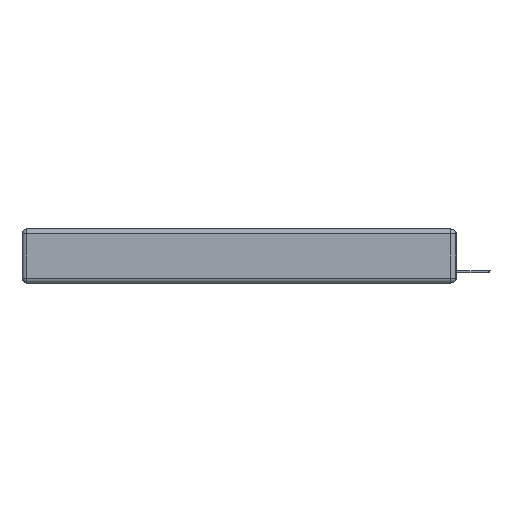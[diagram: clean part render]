
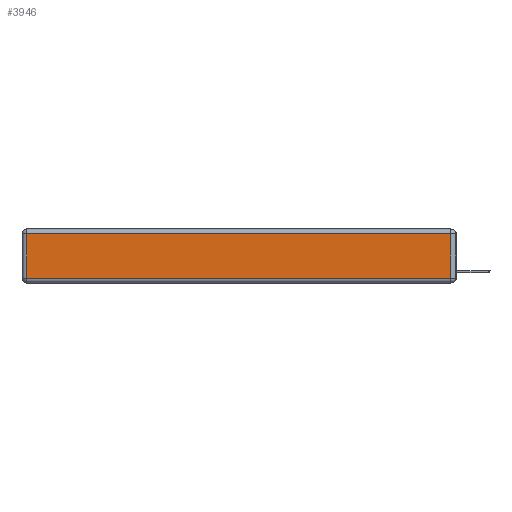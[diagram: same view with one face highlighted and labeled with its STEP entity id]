
A CAD part, left-side view. The second image highlights one B-rep face of the part: STEP entity #3946.
In plain terms, the highlighted planar face has unit normal (-1, 0, 0).
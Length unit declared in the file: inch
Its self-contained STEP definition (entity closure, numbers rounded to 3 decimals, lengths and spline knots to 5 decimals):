
#517 = DIRECTION ( 'NONE',  ( 0., 1., 0. ) ) ;
#1067 = VERTEX_POINT ( 'NONE', #14032 ) ;
#1419 = EDGE_LOOP ( 'NONE', ( #9981, #1592, #5271, #12436 ) ) ;
#1592 = ORIENTED_EDGE ( 'NONE', *, *, #12692, .T. ) ;
#1711 = EDGE_CURVE ( 'NONE', #8032, #10119, #11388, .T. ) ;
#3587 = LINE ( 'NONE', #9226, #16552 ) ;
#3635 = CARTESIAN_POINT ( 'NONE',  ( 0., 2.72, -0.03 ) ) ;
#3847 = CARTESIAN_POINT ( 'NONE',  ( 0., 0.03, -0.313 ) ) ;
#3946 = ADVANCED_FACE ( 'NONE', ( #14470 ), #17246, .T. ) ;
#4474 = EDGE_CURVE ( 'NONE', #1067, #8032, #13152, .T. ) ;
#4780 = DIRECTION ( 'NONE',  ( 0., -1., 0. ) ) ;
#5271 = ORIENTED_EDGE ( 'NONE', *, *, #4474, .T. ) ;
#5596 = VECTOR ( 'NONE', #517, 39.37008 ) ;
#5714 = EDGE_CURVE ( 'NONE', #10119, #10788, #12902, .T. ) ;
#5814 = CARTESIAN_POINT ( 'NONE',  ( 0., 2.72, -0.313 ) ) ;
#8032 = VERTEX_POINT ( 'NONE', #3635 ) ;
#9008 = CARTESIAN_POINT ( 'NONE',  ( 0., 2.75, -0.03 ) ) ;
#9226 = CARTESIAN_POINT ( 'NONE',  ( 0., 0.03, -0.343 ) ) ;
#9981 = ORIENTED_EDGE ( 'NONE', *, *, #5714, .T. ) ;
#10119 = VERTEX_POINT ( 'NONE', #5814 ) ;
#10250 = DIRECTION ( 'NONE',  ( 0., 0., 1. ) ) ;
#10788 = VERTEX_POINT ( 'NONE', #3847 ) ;
#11388 = LINE ( 'NONE', #15809, #14341 ) ;
#11525 = CARTESIAN_POINT ( 'NONE',  ( 0., 0., -0.313 ) ) ;
#12436 = ORIENTED_EDGE ( 'NONE', *, *, #1711, .T. ) ;
#12692 = EDGE_CURVE ( 'NONE', #10788, #1067, #3587, .T. ) ;
#12778 = DIRECTION ( 'NONE',  ( 0., 0., -1. ) ) ;
#12902 = LINE ( 'NONE', #11525, #16504 ) ;
#13018 = CARTESIAN_POINT ( 'NONE',  ( 0., 0., -0.343 ) ) ;
#13152 = LINE ( 'NONE', #9008, #5596 ) ;
#13896 = DIRECTION ( 'NONE',  ( 0., 0., 1. ) ) ;
#14032 = CARTESIAN_POINT ( 'NONE',  ( 0., 0.03, -0.03 ) ) ;
#14341 = VECTOR ( 'NONE', #12778, 39.37008 ) ;
#14470 = FACE_OUTER_BOUND ( 'NONE', #1419, .T. ) ;
#15774 = DIRECTION ( 'NONE',  ( -1., 0., 0. ) ) ;
#15809 = CARTESIAN_POINT ( 'NONE',  ( 0., 2.72, -0.343 ) ) ;
#16504 = VECTOR ( 'NONE', #4780, 39.37008 ) ;
#16552 = VECTOR ( 'NONE', #13896, 39.37008 ) ;
#17246 = PLANE ( 'NONE',  #17699 ) ;
#17699 = AXIS2_PLACEMENT_3D ( 'NONE', #13018, #15774, #10250 ) ;
